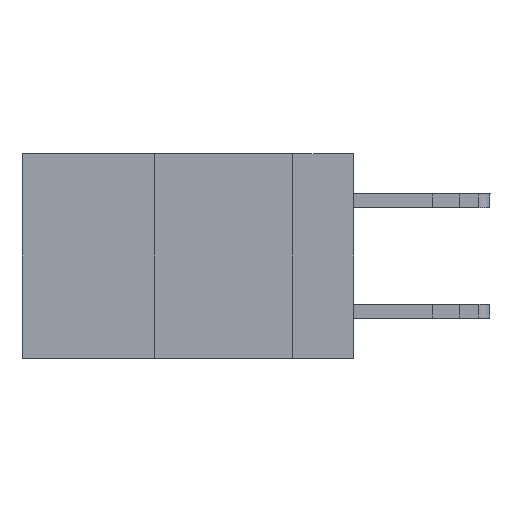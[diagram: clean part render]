
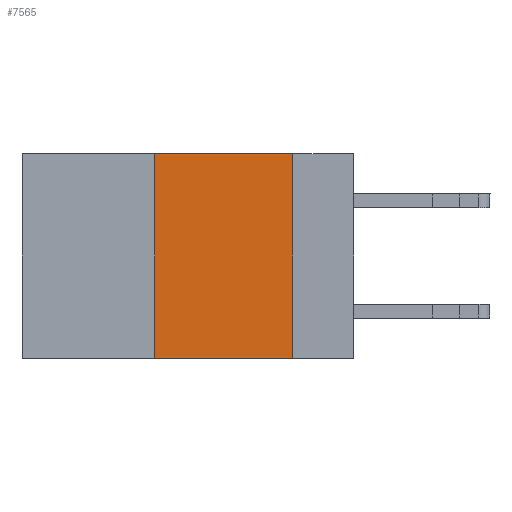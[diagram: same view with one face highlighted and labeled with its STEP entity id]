
A CAD part, left-side view. The second image highlights one B-rep face of the part: STEP entity #7565.
In plain terms, the highlighted planar face has unit normal (-1, 0, 0).
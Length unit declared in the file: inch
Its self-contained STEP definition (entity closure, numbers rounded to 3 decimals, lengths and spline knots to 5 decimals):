
#60 = ORIENTED_EDGE ( 'NONE', *, *, #16477, .F. ) ;
#1876 = LINE ( 'NONE', #5714, #14493 ) ;
#4127 = DIRECTION ( 'NONE',  ( 1., 0., 0. ) ) ;
#4155 = CARTESIAN_POINT ( 'NONE',  ( 0., 0.36, -0.37 ) ) ;
#4605 = FACE_OUTER_BOUND ( 'NONE', #18343, .T. ) ;
#5125 = CARTESIAN_POINT ( 'NONE',  ( 0., 0.11, -0.37 ) ) ;
#5680 = VECTOR ( 'NONE', #11915, 39.37008 ) ;
#5714 = CARTESIAN_POINT ( 'NONE',  ( 0., 0.11, 0. ) ) ;
#6918 = ORIENTED_EDGE ( 'NONE', *, *, #15540, .F. ) ;
#7009 = VERTEX_POINT ( 'NONE', #10035 ) ;
#7565 = ADVANCED_FACE ( 'NONE', ( #4605 ), #14413, .F. ) ;
#8428 = CARTESIAN_POINT ( 'NONE',  ( 0., 0.6, 0. ) ) ;
#8642 = DIRECTION ( 'NONE',  ( 0., 0., -1. ) ) ;
#9534 = CARTESIAN_POINT ( 'NONE',  ( 0., 0.6, 0. ) ) ;
#9718 = EDGE_CURVE ( 'NONE', #7009, #19351, #18558, .T. ) ;
#9797 = DIRECTION ( 'NONE',  ( 0., -1., 0. ) ) ;
#10035 = CARTESIAN_POINT ( 'NONE',  ( 0., 0.36, 0. ) ) ;
#11915 = DIRECTION ( 'NONE',  ( 0., -1., 0. ) ) ;
#12240 = CARTESIAN_POINT ( 'NONE',  ( 0., 0.36, 0. ) ) ;
#13562 = VERTEX_POINT ( 'NONE', #4155 ) ;
#14112 = EDGE_CURVE ( 'NONE', #13562, #16342, #14312, .T. ) ;
#14312 = LINE ( 'NONE', #19348, #5680 ) ;
#14413 = PLANE ( 'NONE',  #16427 ) ;
#14493 = VECTOR ( 'NONE', #19023, 39.37008 ) ;
#14593 = VECTOR ( 'NONE', #9797, 39.37008 ) ;
#14733 = ORIENTED_EDGE ( 'NONE', *, *, #14112, .T. ) ;
#14780 = CARTESIAN_POINT ( 'NONE',  ( 0., 0.11, 0. ) ) ;
#15129 = VECTOR ( 'NONE', #15506, 39.37008 ) ;
#15506 = DIRECTION ( 'NONE',  ( 0., 0., 1. ) ) ;
#15540 = EDGE_CURVE ( 'NONE', #19351, #16342, #1876, .T. ) ;
#16057 = LINE ( 'NONE', #12240, #15129 ) ;
#16342 = VERTEX_POINT ( 'NONE', #5125 ) ;
#16427 = AXIS2_PLACEMENT_3D ( 'NONE', #8428, #4127, #8642 ) ;
#16477 = EDGE_CURVE ( 'NONE', #13562, #7009, #16057, .T. ) ;
#17740 = ORIENTED_EDGE ( 'NONE', *, *, #9718, .F. ) ;
#18343 = EDGE_LOOP ( 'NONE', ( #6918, #17740, #60, #14733 ) ) ;
#18558 = LINE ( 'NONE', #9534, #14593 ) ;
#19023 = DIRECTION ( 'NONE',  ( 0., 0., -1. ) ) ;
#19348 = CARTESIAN_POINT ( 'NONE',  ( 0., 0.6, -0.37 ) ) ;
#19351 = VERTEX_POINT ( 'NONE', #14780 ) ;
